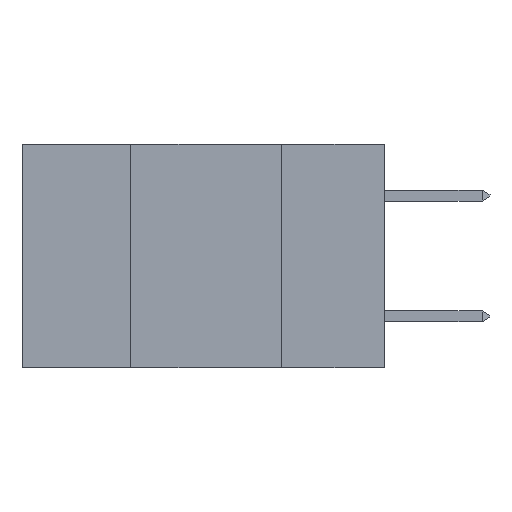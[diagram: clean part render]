
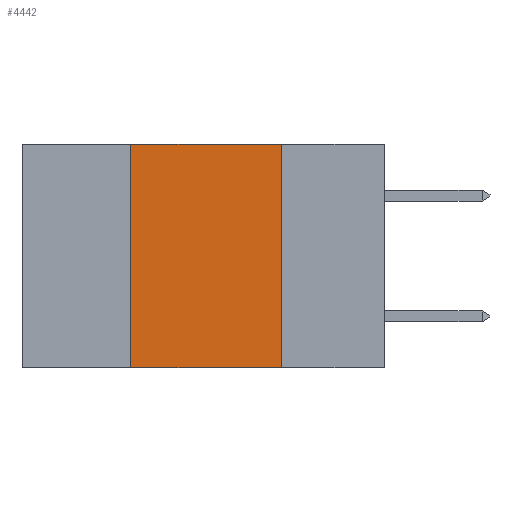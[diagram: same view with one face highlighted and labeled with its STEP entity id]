
A CAD part, left-side view. The second image highlights one B-rep face of the part: STEP entity #4442.
In plain terms, the highlighted planar face has unit normal (-1, 0, 0).
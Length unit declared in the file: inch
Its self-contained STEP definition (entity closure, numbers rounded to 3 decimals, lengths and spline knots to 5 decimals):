
#421 = CARTESIAN_POINT ( 'NONE',  ( 0., 0.42, 0. ) ) ;
#958 = DIRECTION ( 'NONE',  ( 0., -1., 0. ) ) ;
#1787 = VERTEX_POINT ( 'NONE', #421 ) ;
#2085 = ORIENTED_EDGE ( 'NONE', *, *, #7908, .F. ) ;
#2869 = DIRECTION ( 'NONE',  ( 0., 0., 1. ) ) ;
#3024 = DIRECTION ( 'NONE',  ( 0., -1., 0. ) ) ;
#3281 = CARTESIAN_POINT ( 'NONE',  ( 0., 0.6, -0.37 ) ) ;
#3512 = DIRECTION ( 'NONE',  ( 0., 0., -1. ) ) ;
#3948 = VECTOR ( 'NONE', #16535, 39.37008 ) ;
#4442 = ADVANCED_FACE ( 'NONE', ( #7038 ), #8931, .F. ) ;
#4981 = EDGE_LOOP ( 'NONE', ( #2085, #12351, #13821, #6537 ) ) ;
#5237 = VECTOR ( 'NONE', #958, 39.37008 ) ;
#5513 = VECTOR ( 'NONE', #3024, 39.37008 ) ;
#6025 = EDGE_CURVE ( 'NONE', #8578, #7356, #9090, .T. ) ;
#6097 = AXIS2_PLACEMENT_3D ( 'NONE', #13011, #17008, #3512 ) ;
#6537 = ORIENTED_EDGE ( 'NONE', *, *, #6025, .T. ) ;
#6807 = EDGE_CURVE ( 'NONE', #8578, #1787, #13938, .T. ) ;
#7038 = FACE_OUTER_BOUND ( 'NONE', #4981, .T. ) ;
#7356 = VERTEX_POINT ( 'NONE', #14525 ) ;
#7537 = CARTESIAN_POINT ( 'NONE',  ( 0., 0.17, 0. ) ) ;
#7599 = EDGE_CURVE ( 'NONE', #1787, #9805, #13701, .T. ) ;
#7908 = EDGE_CURVE ( 'NONE', #9805, #7356, #15595, .T. ) ;
#8578 = VERTEX_POINT ( 'NONE', #9461 ) ;
#8931 = PLANE ( 'NONE',  #6097 ) ;
#9090 = LINE ( 'NONE', #3281, #5513 ) ;
#9461 = CARTESIAN_POINT ( 'NONE',  ( 0., 0.42, -0.37 ) ) ;
#9805 = VERTEX_POINT ( 'NONE', #7537 ) ;
#10525 = CARTESIAN_POINT ( 'NONE',  ( 0., 0.6, 0. ) ) ;
#11096 = CARTESIAN_POINT ( 'NONE',  ( 0., 0.42, 0. ) ) ;
#12351 = ORIENTED_EDGE ( 'NONE', *, *, #7599, .F. ) ;
#12448 = CARTESIAN_POINT ( 'NONE',  ( 0., 0.17, 0. ) ) ;
#13011 = CARTESIAN_POINT ( 'NONE',  ( 0., 0.6, 0. ) ) ;
#13701 = LINE ( 'NONE', #10525, #5237 ) ;
#13821 = ORIENTED_EDGE ( 'NONE', *, *, #6807, .F. ) ;
#13938 = LINE ( 'NONE', #11096, #16082 ) ;
#14525 = CARTESIAN_POINT ( 'NONE',  ( 0., 0.17, -0.37 ) ) ;
#15595 = LINE ( 'NONE', #12448, #3948 ) ;
#16082 = VECTOR ( 'NONE', #2869, 39.37008 ) ;
#16535 = DIRECTION ( 'NONE',  ( 0., 0., -1. ) ) ;
#17008 = DIRECTION ( 'NONE',  ( 1., 0., 0. ) ) ;
